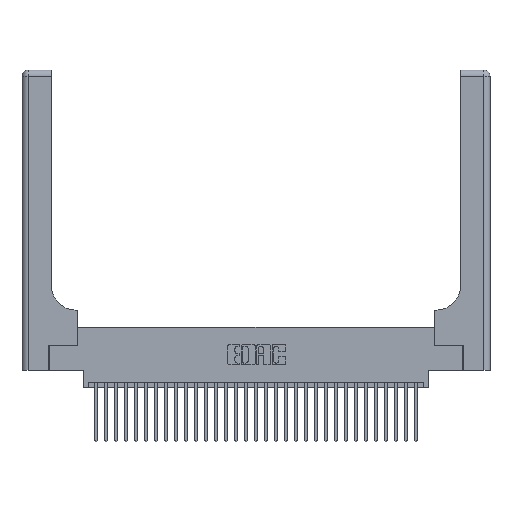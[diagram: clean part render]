
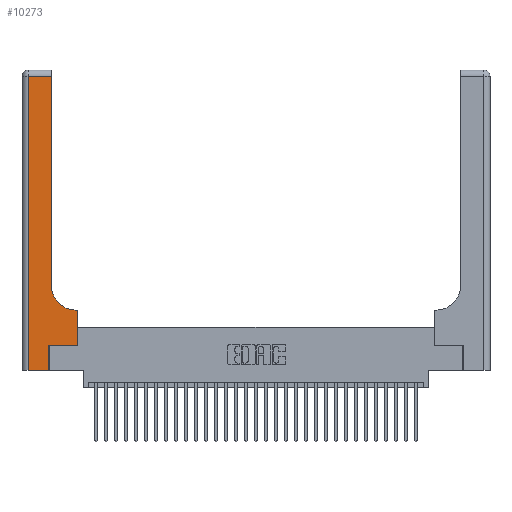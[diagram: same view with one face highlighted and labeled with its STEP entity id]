
A CAD part, top view. The second image highlights one B-rep face of the part: STEP entity #10273.
In plain terms, the highlighted planar face has unit normal (0, 0, 1).
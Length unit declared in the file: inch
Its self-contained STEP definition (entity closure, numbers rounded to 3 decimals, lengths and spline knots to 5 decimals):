
#1036 = VERTEX_POINT ( 'NONE', #24259 ) ;
#1276 = LINE ( 'NONE', #6921, #5556 ) ;
#1610 = DIRECTION ( 'NONE',  ( 1., 0., 0. ) ) ;
#1951 = VECTOR ( 'NONE', #15534, 39.37008 ) ;
#2131 = ORIENTED_EDGE ( 'NONE', *, *, #28427, .T. ) ;
#2383 = LINE ( 'NONE', #28294, #3158 ) ;
#2463 = CARTESIAN_POINT ( 'NONE',  ( 0.2915, 0.6, 0.37 ) ) ;
#3158 = VECTOR ( 'NONE', #5912, 39.37008 ) ;
#3639 = EDGE_CURVE ( 'NONE', #28070, #22311, #22737, .T. ) ;
#4597 = VECTOR ( 'NONE', #28028, 39.37008 ) ;
#4930 = ORIENTED_EDGE ( 'NONE', *, *, #16730, .T. ) ;
#5390 = VERTEX_POINT ( 'NONE', #21570 ) ;
#5493 = VERTEX_POINT ( 'NONE', #7596 ) ;
#5556 = VECTOR ( 'NONE', #6807, 39.37008 ) ;
#5652 = EDGE_CURVE ( 'NONE', #22311, #16072, #32066, .T. ) ;
#5912 = DIRECTION ( 'NONE',  ( 1., 0., 0. ) ) ;
#6807 = DIRECTION ( 'NONE',  ( 0., 1., 0. ) ) ;
#6921 = CARTESIAN_POINT ( 'NONE',  ( 0.2915, 3., 0.37 ) ) ;
#7416 = ORIENTED_EDGE ( 'NONE', *, *, #3639, .T. ) ;
#7592 = VERTEX_POINT ( 'NONE', #11721 ) ;
#7596 = CARTESIAN_POINT ( 'NONE',  ( 0.2915, 2.94, 0.37 ) ) ;
#8144 = CARTESIAN_POINT ( 'NONE',  ( 0., 0., 0.37 ) ) ;
#9135 = FACE_OUTER_BOUND ( 'NONE', #13387, .T. ) ;
#9175 = CARTESIAN_POINT ( 'NONE',  ( 0.5415, 0.85, 0.37 ) ) ;
#9420 = CARTESIAN_POINT ( 'NONE',  ( 0.269, 0., 0.37 ) ) ;
#10273 = ADVANCED_FACE ( 'NONE', ( #9135 ), #11702, .F. ) ;
#10316 = VECTOR ( 'NONE', #17885, 39.37008 ) ;
#10361 = CARTESIAN_POINT ( 'NONE',  ( 0.5585, 0.25, 0.37 ) ) ;
#11246 = LINE ( 'NONE', #10361, #21840 ) ;
#11414 = EDGE_CURVE ( 'NONE', #15316, #5493, #1276, .T. ) ;
#11702 = PLANE ( 'NONE',  #26390 ) ;
#11721 = CARTESIAN_POINT ( 'NONE',  ( 0.5585, 0.6, 0.37 ) ) ;
#13387 = EDGE_LOOP ( 'NONE', ( #23689, #17440, #31930, #7416, #31500, #20480, #4930, #26302, #2131 ) ) ;
#14271 = CARTESIAN_POINT ( 'NONE',  ( 0.269, 0., 0.37 ) ) ;
#15316 = VERTEX_POINT ( 'NONE', #21551 ) ;
#15534 = DIRECTION ( 'NONE',  ( 1., 0., 0. ) ) ;
#15883 = VECTOR ( 'NONE', #22838, 39.37008 ) ;
#16072 = VERTEX_POINT ( 'NONE', #24164 ) ;
#16607 = VERTEX_POINT ( 'NONE', #21917 ) ;
#16730 = EDGE_CURVE ( 'NONE', #5390, #7592, #11246, .T. ) ;
#16888 = CARTESIAN_POINT ( 'NONE',  ( 0., 3., 0.37 ) ) ;
#17031 = LINE ( 'NONE', #17985, #10316 ) ;
#17381 = AXIS2_PLACEMENT_3D ( 'NONE', #9175, #31666, #1610 ) ;
#17440 = ORIENTED_EDGE ( 'NONE', *, *, #30532, .T. ) ;
#17885 = DIRECTION ( 'NONE',  ( -1., 0., 0. ) ) ;
#17985 = CARTESIAN_POINT ( 'NONE',  ( 0., 2.94, 0.37 ) ) ;
#18941 = DIRECTION ( 'NONE',  ( 0., -1., 0. ) ) ;
#20037 = CARTESIAN_POINT ( 'NONE',  ( 0.06, 0., 0.37 ) ) ;
#20312 = DIRECTION ( 'NONE',  ( 0., 1., 0. ) ) ;
#20325 = EDGE_CURVE ( 'NONE', #1036, #28070, #24808, .T. ) ;
#20480 = ORIENTED_EDGE ( 'NONE', *, *, #25615, .T. ) ;
#20861 = VECTOR ( 'NONE', #18941, 39.37008 ) ;
#21551 = CARTESIAN_POINT ( 'NONE',  ( 0.2915, 0.85, 0.37 ) ) ;
#21570 = CARTESIAN_POINT ( 'NONE',  ( 0.5585, 0.25, 0.37 ) ) ;
#21730 = LINE ( 'NONE', #2463, #15883 ) ;
#21840 = VECTOR ( 'NONE', #20312, 39.37008 ) ;
#21917 = CARTESIAN_POINT ( 'NONE',  ( 0.5415, 0.6, 0.37 ) ) ;
#22311 = VERTEX_POINT ( 'NONE', #14271 ) ;
#22737 = LINE ( 'NONE', #8144, #1951 ) ;
#22838 = DIRECTION ( 'NONE',  ( -1., 0., 0. ) ) ;
#22901 = EDGE_CURVE ( 'NONE', #7592, #16607, #21730, .T. ) ;
#23057 = CIRCLE ( 'NONE', #17381, 0.25 ) ;
#23689 = ORIENTED_EDGE ( 'NONE', *, *, #11414, .T. ) ;
#24089 = CARTESIAN_POINT ( 'NONE',  ( 0.06, 3., 0.37 ) ) ;
#24164 = CARTESIAN_POINT ( 'NONE',  ( 0.269, 0.25, 0.37 ) ) ;
#24259 = CARTESIAN_POINT ( 'NONE',  ( 0.06, 2.94, 0.37 ) ) ;
#24808 = LINE ( 'NONE', #24089, #20861 ) ;
#25615 = EDGE_CURVE ( 'NONE', #16072, #5390, #2383, .T. ) ;
#26302 = ORIENTED_EDGE ( 'NONE', *, *, #22901, .T. ) ;
#26390 = AXIS2_PLACEMENT_3D ( 'NONE', #16888, #26948, #27057 ) ;
#26948 = DIRECTION ( 'NONE',  ( 0., 0., -1. ) ) ;
#27057 = DIRECTION ( 'NONE',  ( -1., 0., 0. ) ) ;
#28028 = DIRECTION ( 'NONE',  ( 0., 1., 0. ) ) ;
#28070 = VERTEX_POINT ( 'NONE', #20037 ) ;
#28294 = CARTESIAN_POINT ( 'NONE',  ( 0.269, 0.25, 0.37 ) ) ;
#28427 = EDGE_CURVE ( 'NONE', #16607, #15316, #23057, .T. ) ;
#30532 = EDGE_CURVE ( 'NONE', #5493, #1036, #17031, .T. ) ;
#31500 = ORIENTED_EDGE ( 'NONE', *, *, #5652, .T. ) ;
#31666 = DIRECTION ( 'NONE',  ( 0., 0., -1. ) ) ;
#31930 = ORIENTED_EDGE ( 'NONE', *, *, #20325, .T. ) ;
#32066 = LINE ( 'NONE', #9420, #4597 ) ;
